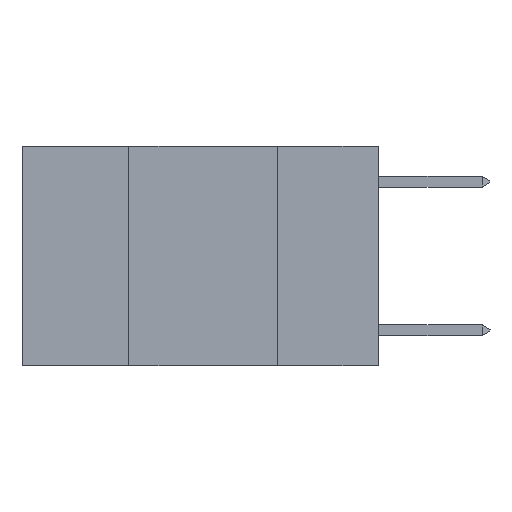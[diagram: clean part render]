
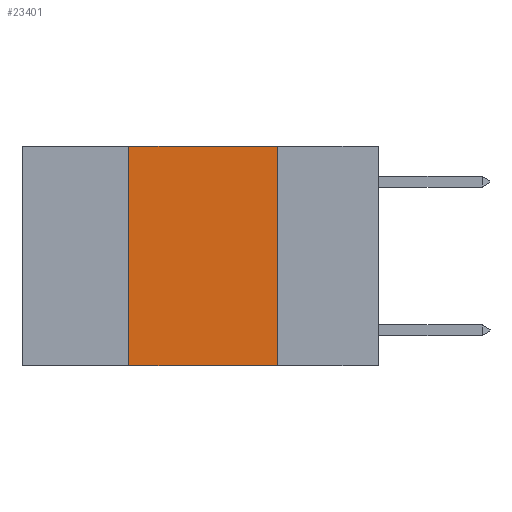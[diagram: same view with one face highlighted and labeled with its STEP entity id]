
A CAD part, left-side view. The second image highlights one B-rep face of the part: STEP entity #23401.
In plain terms, the highlighted planar face has unit normal (-1, 0, 0).
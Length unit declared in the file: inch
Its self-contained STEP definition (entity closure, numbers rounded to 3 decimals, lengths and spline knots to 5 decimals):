
#627 = EDGE_CURVE ( 'NONE', #27103, #24776, #30725, .T. ) ;
#632 = CARTESIAN_POINT ( 'NONE',  ( 0., 0.17, 0. ) ) ;
#689 = ORIENTED_EDGE ( 'NONE', *, *, #27528, .T. ) ;
#1691 = VECTOR ( 'NONE', #26327, 39.37008 ) ;
#1924 = DIRECTION ( 'NONE',  ( 0., -1., 0. ) ) ;
#3964 = DIRECTION ( 'NONE',  ( 0., 0., -1. ) ) ;
#4389 = VECTOR ( 'NONE', #1924, 39.37008 ) ;
#4665 = CARTESIAN_POINT ( 'NONE',  ( 0., 0.42, 0. ) ) ;
#5294 = CARTESIAN_POINT ( 'NONE',  ( 0., 0.17, -0.37 ) ) ;
#7441 = LINE ( 'NONE', #17413, #28348 ) ;
#7461 = CARTESIAN_POINT ( 'NONE',  ( 0., 0.42, 0. ) ) ;
#9434 = CARTESIAN_POINT ( 'NONE',  ( 0., 0.6, 0. ) ) ;
#9959 = VERTEX_POINT ( 'NONE', #4665 ) ;
#10990 = CARTESIAN_POINT ( 'NONE',  ( 0., 0.6, 0. ) ) ;
#11874 = VERTEX_POINT ( 'NONE', #29361 ) ;
#12541 = ORIENTED_EDGE ( 'NONE', *, *, #28521, .F. ) ;
#13089 = EDGE_CURVE ( 'NONE', #11874, #9959, #17109, .T. ) ;
#17109 = LINE ( 'NONE', #7461, #23534 ) ;
#17413 = CARTESIAN_POINT ( 'NONE',  ( 0., 0.6, -0.37 ) ) ;
#20047 = DIRECTION ( 'NONE',  ( 0., 0., 1. ) ) ;
#23263 = DIRECTION ( 'NONE',  ( 1., 0., 0. ) ) ;
#23401 = ADVANCED_FACE ( 'NONE', ( #31399 ), #23420, .F. ) ;
#23420 = PLANE ( 'NONE',  #25648 ) ;
#23529 = ORIENTED_EDGE ( 'NONE', *, *, #627, .F. ) ;
#23534 = VECTOR ( 'NONE', #20047, 39.37008 ) ;
#24776 = VERTEX_POINT ( 'NONE', #5294 ) ;
#25648 = AXIS2_PLACEMENT_3D ( 'NONE', #10990, #23263, #3964 ) ;
#26007 = CARTESIAN_POINT ( 'NONE',  ( 0., 0.17, 0. ) ) ;
#26327 = DIRECTION ( 'NONE',  ( 0., 0., -1. ) ) ;
#27103 = VERTEX_POINT ( 'NONE', #632 ) ;
#27391 = DIRECTION ( 'NONE',  ( 0., -1., 0. ) ) ;
#27528 = EDGE_CURVE ( 'NONE', #11874, #24776, #7441, .T. ) ;
#28348 = VECTOR ( 'NONE', #27391, 39.37008 ) ;
#28521 = EDGE_CURVE ( 'NONE', #9959, #27103, #29217, .T. ) ;
#29217 = LINE ( 'NONE', #9434, #4389 ) ;
#29361 = CARTESIAN_POINT ( 'NONE',  ( 0., 0.42, -0.37 ) ) ;
#30725 = LINE ( 'NONE', #26007, #1691 ) ;
#31264 = EDGE_LOOP ( 'NONE', ( #23529, #12541, #32175, #689 ) ) ;
#31399 = FACE_OUTER_BOUND ( 'NONE', #31264, .T. ) ;
#32175 = ORIENTED_EDGE ( 'NONE', *, *, #13089, .F. ) ;
